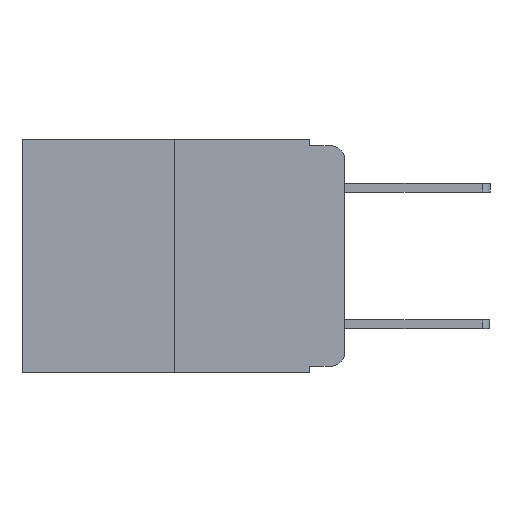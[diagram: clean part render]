
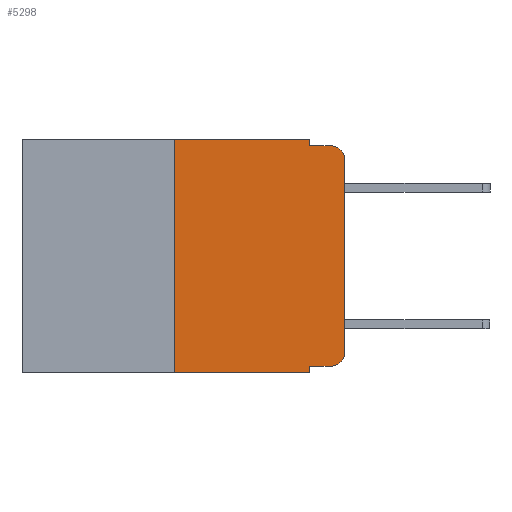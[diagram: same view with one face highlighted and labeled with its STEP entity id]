
A CAD part, left-side view. The second image highlights one B-rep face of the part: STEP entity #5298.
In plain terms, the highlighted planar face has unit normal (-1, 0, 0).
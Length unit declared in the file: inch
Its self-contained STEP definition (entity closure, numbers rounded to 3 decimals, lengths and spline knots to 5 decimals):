
#235 = PLANE ( 'NONE',  #3060 ) ;
#405 = FACE_OUTER_BOUND ( 'NONE', #6678, .T. ) ;
#525 = VECTOR ( 'NONE', #10231, 39.37008 ) ;
#818 = LINE ( 'NONE', #7699, #4283 ) ;
#1069 = VECTOR ( 'NONE', #6330, 39.37008 ) ;
#1360 = DIRECTION ( 'NONE',  ( 0., 0., -1. ) ) ;
#1552 = EDGE_CURVE ( 'NONE', #12409, #15097, #6741, .T. ) ;
#1661 = VERTEX_POINT ( 'NONE', #9568 ) ;
#1741 = CARTESIAN_POINT ( 'NONE',  ( 0., 0.051, -0.333 ) ) ;
#1900 = VERTEX_POINT ( 'NONE', #3027 ) ;
#2014 = ORIENTED_EDGE ( 'NONE', *, *, #12999, .F. ) ;
#2219 = ORIENTED_EDGE ( 'NONE', *, *, #2546, .F. ) ;
#2457 = VERTEX_POINT ( 'NONE', #5716 ) ;
#2546 = EDGE_CURVE ( 'NONE', #15097, #14514, #4680, .T. ) ;
#2924 = CARTESIAN_POINT ( 'NONE',  ( 0., 0.051, -0.01 ) ) ;
#2940 = ORIENTED_EDGE ( 'NONE', *, *, #4538, .T. ) ;
#3027 = CARTESIAN_POINT ( 'NONE',  ( 0., 0.02, -0.333 ) ) ;
#3060 = AXIS2_PLACEMENT_3D ( 'NONE', #3093, #3169, #12708 ) ;
#3093 = CARTESIAN_POINT ( 'NONE',  ( 0., 0.473, 0. ) ) ;
#3169 = DIRECTION ( 'NONE',  ( 1., 0., 0. ) ) ;
#3401 = CARTESIAN_POINT ( 'NONE',  ( 0., 0.051, -0.333 ) ) ;
#3542 = EDGE_CURVE ( 'NONE', #12872, #14514, #11884, .T. ) ;
#3563 = LINE ( 'NONE', #10554, #6925 ) ;
#3684 = DIRECTION ( 'NONE',  ( 0., 0., 1. ) ) ;
#4053 = VERTEX_POINT ( 'NONE', #11408 ) ;
#4283 = VECTOR ( 'NONE', #6305, 39.37008 ) ;
#4538 = EDGE_CURVE ( 'NONE', #1661, #12872, #4907, .T. ) ;
#4680 = LINE ( 'NONE', #6543, #7971 ) ;
#4862 = CARTESIAN_POINT ( 'NONE',  ( 0., 0.473, -0.343 ) ) ;
#4907 = LINE ( 'NONE', #7595, #525 ) ;
#4918 = DIRECTION ( 'NONE',  ( 0., -1., 0. ) ) ;
#4925 = EDGE_CURVE ( 'NONE', #2457, #12409, #13857, .T. ) ;
#5198 = ORIENTED_EDGE ( 'NONE', *, *, #10386, .T. ) ;
#5298 = ADVANCED_FACE ( 'NONE', ( #405 ), #235, .F. ) ;
#5452 = VERTEX_POINT ( 'NONE', #9153 ) ;
#5716 = CARTESIAN_POINT ( 'NONE',  ( 0., 0.25, 0. ) ) ;
#6190 = DIRECTION ( 'NONE',  ( 0., -1., 0. ) ) ;
#6256 = DIRECTION ( 'NONE',  ( -1., 0., 0. ) ) ;
#6262 = CARTESIAN_POINT ( 'NONE',  ( 0., 0.02, -0.01 ) ) ;
#6305 = DIRECTION ( 'NONE',  ( 0., 0., -1. ) ) ;
#6330 = DIRECTION ( 'NONE',  ( 0., -1., 0. ) ) ;
#6370 = VECTOR ( 'NONE', #4918, 39.37008 ) ;
#6543 = CARTESIAN_POINT ( 'NONE',  ( 0., 0.051, -0.01 ) ) ;
#6678 = EDGE_LOOP ( 'NONE', ( #2940, #14395, #2219, #14651, #16641, #14292, #13928, #2014, #13140, #5198 ) ) ;
#6741 = LINE ( 'NONE', #9447, #13898 ) ;
#6925 = VECTOR ( 'NONE', #3684, 39.37008 ) ;
#7122 = AXIS2_PLACEMENT_3D ( 'NONE', #17408, #9809, #1360 ) ;
#7567 = DIRECTION ( 'NONE',  ( 0., -1., 0. ) ) ;
#7595 = CARTESIAN_POINT ( 'NONE',  ( 0., 0., 0. ) ) ;
#7699 = CARTESIAN_POINT ( 'NONE',  ( 0., 0.051, 0. ) ) ;
#7971 = VECTOR ( 'NONE', #6190, 39.37008 ) ;
#8692 = VERTEX_POINT ( 'NONE', #1741 ) ;
#9153 = CARTESIAN_POINT ( 'NONE',  ( 0., 0.25, -0.343 ) ) ;
#9382 = DIRECTION ( 'NONE',  ( 0., 0., -1. ) ) ;
#9447 = CARTESIAN_POINT ( 'NONE',  ( 0., 0.051, 0. ) ) ;
#9550 = CIRCLE ( 'NONE', #15475, 0.02 ) ;
#9568 = CARTESIAN_POINT ( 'NONE',  ( 0., 0., -0.313 ) ) ;
#9809 = DIRECTION ( 'NONE',  ( -1., 0., 0. ) ) ;
#9920 = LINE ( 'NONE', #4862, #6370 ) ;
#10231 = DIRECTION ( 'NONE',  ( 0., 0., 1. ) ) ;
#10386 = EDGE_CURVE ( 'NONE', #1900, #1661, #9550, .T. ) ;
#10426 = VECTOR ( 'NONE', #7567, 39.37008 ) ;
#10554 = CARTESIAN_POINT ( 'NONE',  ( 0., 0.25, 0. ) ) ;
#11408 = CARTESIAN_POINT ( 'NONE',  ( 0., 0.051, -0.343 ) ) ;
#11476 = CARTESIAN_POINT ( 'NONE',  ( 0., 0., -0.03 ) ) ;
#11884 = CIRCLE ( 'NONE', #7122, 0.02 ) ;
#12133 = EDGE_CURVE ( 'NONE', #8692, #1900, #15530, .T. ) ;
#12409 = VERTEX_POINT ( 'NONE', #15803 ) ;
#12708 = DIRECTION ( 'NONE',  ( 0., 0., -1. ) ) ;
#12872 = VERTEX_POINT ( 'NONE', #11476 ) ;
#12999 = EDGE_CURVE ( 'NONE', #8692, #4053, #818, .T. ) ;
#13140 = ORIENTED_EDGE ( 'NONE', *, *, #12133, .T. ) ;
#13840 = EDGE_CURVE ( 'NONE', #5452, #2457, #3563, .T. ) ;
#13857 = LINE ( 'NONE', #16550, #10426 ) ;
#13898 = VECTOR ( 'NONE', #9382, 39.37008 ) ;
#13928 = ORIENTED_EDGE ( 'NONE', *, *, #17359, .T. ) ;
#14141 = CARTESIAN_POINT ( 'NONE',  ( 0., 0.02, -0.313 ) ) ;
#14292 = ORIENTED_EDGE ( 'NONE', *, *, #13840, .F. ) ;
#14395 = ORIENTED_EDGE ( 'NONE', *, *, #3542, .T. ) ;
#14514 = VERTEX_POINT ( 'NONE', #6262 ) ;
#14651 = ORIENTED_EDGE ( 'NONE', *, *, #1552, .F. ) ;
#15097 = VERTEX_POINT ( 'NONE', #2924 ) ;
#15387 = DIRECTION ( 'NONE',  ( 0., 0., -1. ) ) ;
#15475 = AXIS2_PLACEMENT_3D ( 'NONE', #14141, #6256, #15387 ) ;
#15530 = LINE ( 'NONE', #3401, #1069 ) ;
#15803 = CARTESIAN_POINT ( 'NONE',  ( 0., 0.051, 0. ) ) ;
#16550 = CARTESIAN_POINT ( 'NONE',  ( 0., 0.473, 0. ) ) ;
#16641 = ORIENTED_EDGE ( 'NONE', *, *, #4925, .F. ) ;
#17359 = EDGE_CURVE ( 'NONE', #5452, #4053, #9920, .T. ) ;
#17408 = CARTESIAN_POINT ( 'NONE',  ( 0., 0.02, -0.03 ) ) ;
